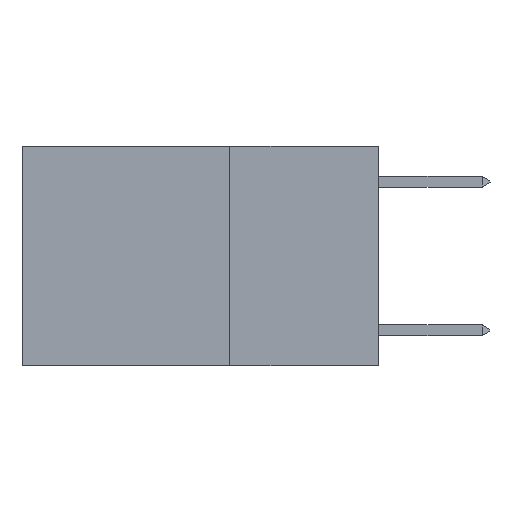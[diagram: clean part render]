
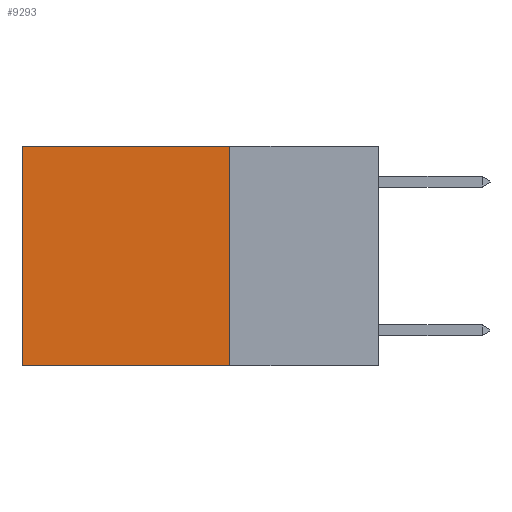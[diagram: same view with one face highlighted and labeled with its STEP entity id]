
A CAD part, left-side view. The second image highlights one B-rep face of the part: STEP entity #9293.
In plain terms, the highlighted planar face has unit normal (-1, 0, 0).
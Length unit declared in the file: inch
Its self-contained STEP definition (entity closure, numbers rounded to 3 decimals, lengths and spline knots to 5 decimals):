
#2 = VECTOR ( 'NONE', #6106, 39.37008 ) ;
#285 = DIRECTION ( 'NONE',  ( 0., 1., 0. ) ) ;
#759 = CARTESIAN_POINT ( 'NONE',  ( 0.2625, 0.25, 0. ) ) ;
#912 = LINE ( 'NONE', #2581, #2 ) ;
#1190 = ORIENTED_EDGE ( 'NONE', *, *, #21240, .T. ) ;
#1635 = EDGE_LOOP ( 'NONE', ( #16109, #14517, #21124, #1190 ) ) ;
#2218 = DIRECTION ( 'NONE',  ( 0., 1., 0. ) ) ;
#2581 = CARTESIAN_POINT ( 'NONE',  ( 0.2625, 0.25, 0. ) ) ;
#3825 = LINE ( 'NONE', #15832, #12933 ) ;
#4767 = VERTEX_POINT ( 'NONE', #9800 ) ;
#4790 = CARTESIAN_POINT ( 'NONE',  ( 0.2625, 0.6, 0. ) ) ;
#5543 = EDGE_CURVE ( 'NONE', #7892, #17157, #912, .T. ) ;
#5672 = CARTESIAN_POINT ( 'NONE',  ( 0.2625, 0.25, 0. ) ) ;
#5996 = FACE_OUTER_BOUND ( 'NONE', #1635, .T. ) ;
#6106 = DIRECTION ( 'NONE',  ( 0., 0., -1. ) ) ;
#6379 = AXIS2_PLACEMENT_3D ( 'NONE', #5672, #16125, #17758 ) ;
#7552 = CARTESIAN_POINT ( 'NONE',  ( 0.2625, 0.6, 0. ) ) ;
#7706 = LINE ( 'NONE', #759, #15747 ) ;
#7739 = PLANE ( 'NONE',  #6379 ) ;
#7892 = VERTEX_POINT ( 'NONE', #21635 ) ;
#8308 = DIRECTION ( 'NONE',  ( 0., 0., -1. ) ) ;
#9293 = ADVANCED_FACE ( 'NONE', ( #5996 ), #7739, .F. ) ;
#9800 = CARTESIAN_POINT ( 'NONE',  ( 0.2625, 0.6, -0.37 ) ) ;
#10875 = EDGE_CURVE ( 'NONE', #21649, #4767, #16689, .T. ) ;
#11115 = CARTESIAN_POINT ( 'NONE',  ( 0.2625, 0.25, -0.37 ) ) ;
#12933 = VECTOR ( 'NONE', #285, 39.37008 ) ;
#14517 = ORIENTED_EDGE ( 'NONE', *, *, #21499, .F. ) ;
#15747 = VECTOR ( 'NONE', #2218, 39.37008 ) ;
#15832 = CARTESIAN_POINT ( 'NONE',  ( 0.2625, 0.25, -0.37 ) ) ;
#16109 = ORIENTED_EDGE ( 'NONE', *, *, #10875, .T. ) ;
#16125 = DIRECTION ( 'NONE',  ( 1., 0., 0. ) ) ;
#16689 = LINE ( 'NONE', #4790, #20727 ) ;
#17157 = VERTEX_POINT ( 'NONE', #11115 ) ;
#17758 = DIRECTION ( 'NONE',  ( 0., 0., -1. ) ) ;
#20727 = VECTOR ( 'NONE', #8308, 39.37008 ) ;
#21124 = ORIENTED_EDGE ( 'NONE', *, *, #5543, .F. ) ;
#21240 = EDGE_CURVE ( 'NONE', #7892, #21649, #7706, .T. ) ;
#21499 = EDGE_CURVE ( 'NONE', #17157, #4767, #3825, .T. ) ;
#21635 = CARTESIAN_POINT ( 'NONE',  ( 0.2625, 0.25, 0. ) ) ;
#21649 = VERTEX_POINT ( 'NONE', #7552 ) ;
